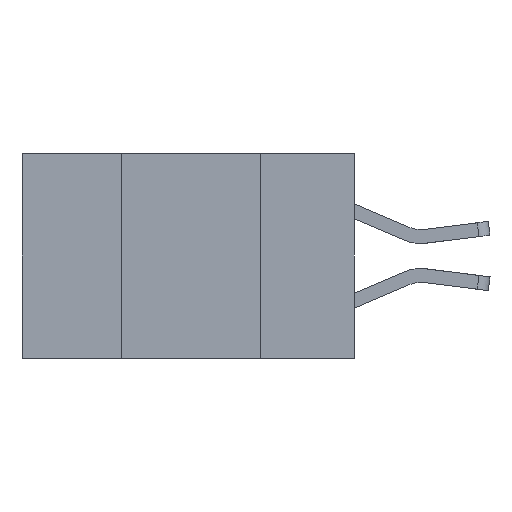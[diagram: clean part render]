
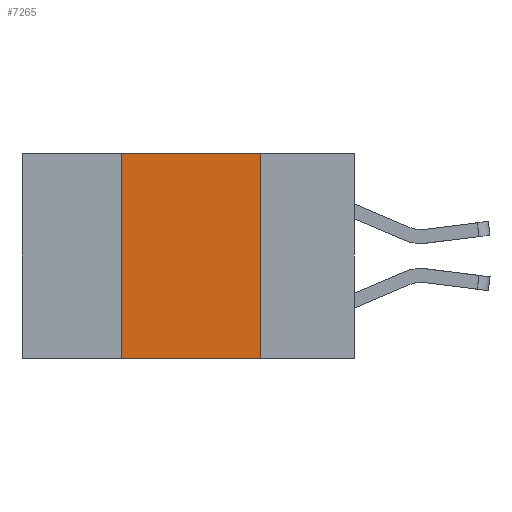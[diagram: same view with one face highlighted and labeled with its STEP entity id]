
A CAD part, left-side view. The second image highlights one B-rep face of the part: STEP entity #7265.
In plain terms, the highlighted planar face has unit normal (-1, 0, 0).
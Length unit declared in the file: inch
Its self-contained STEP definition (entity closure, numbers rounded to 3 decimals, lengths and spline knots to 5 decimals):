
#647 = DIRECTION ( 'NONE',  ( 0., -1., 0. ) ) ;
#957 = EDGE_CURVE ( 'NONE', #5318, #5189, #2652, .T. ) ;
#1039 = PLANE ( 'NONE',  #1068 ) ;
#1068 = AXIS2_PLACEMENT_3D ( 'NONE', #10731, #7375, #2019 ) ;
#1657 = VERTEX_POINT ( 'NONE', #7769 ) ;
#1702 = FACE_OUTER_BOUND ( 'NONE', #4029, .T. ) ;
#1727 = CARTESIAN_POINT ( 'NONE',  ( 0., 0.42, 0. ) ) ;
#1928 = VERTEX_POINT ( 'NONE', #3011 ) ;
#2019 = DIRECTION ( 'NONE',  ( 0., 0., -1. ) ) ;
#2192 = EDGE_CURVE ( 'NONE', #1928, #5189, #9067, .T. ) ;
#2514 = LINE ( 'NONE', #7752, #4333 ) ;
#2652 = LINE ( 'NONE', #10470, #4035 ) ;
#2962 = ORIENTED_EDGE ( 'NONE', *, *, #9389, .F. ) ;
#3011 = CARTESIAN_POINT ( 'NONE',  ( 0., 0.17, 0. ) ) ;
#3498 = DIRECTION ( 'NONE',  ( 0., 0., 1. ) ) ;
#4029 = EDGE_LOOP ( 'NONE', ( #9190, #2962, #11541, #7082 ) ) ;
#4035 = VECTOR ( 'NONE', #8678, 39.37008 ) ;
#4333 = VECTOR ( 'NONE', #647, 39.37008 ) ;
#5189 = VERTEX_POINT ( 'NONE', #11002 ) ;
#5318 = VERTEX_POINT ( 'NONE', #8529 ) ;
#5676 = EDGE_CURVE ( 'NONE', #5318, #1657, #5908, .T. ) ;
#5908 = LINE ( 'NONE', #1727, #10139 ) ;
#6250 = VECTOR ( 'NONE', #7096, 39.37008 ) ;
#7082 = ORIENTED_EDGE ( 'NONE', *, *, #957, .T. ) ;
#7096 = DIRECTION ( 'NONE',  ( 0., 0., -1. ) ) ;
#7265 = ADVANCED_FACE ( 'NONE', ( #1702 ), #1039, .F. ) ;
#7375 = DIRECTION ( 'NONE',  ( 1., 0., 0. ) ) ;
#7752 = CARTESIAN_POINT ( 'NONE',  ( 0., 0.6, 0. ) ) ;
#7769 = CARTESIAN_POINT ( 'NONE',  ( 0., 0.42, 0. ) ) ;
#8529 = CARTESIAN_POINT ( 'NONE',  ( 0., 0.42, -0.37 ) ) ;
#8678 = DIRECTION ( 'NONE',  ( 0., -1., 0. ) ) ;
#8805 = CARTESIAN_POINT ( 'NONE',  ( 0., 0.17, 0. ) ) ;
#9067 = LINE ( 'NONE', #8805, #6250 ) ;
#9190 = ORIENTED_EDGE ( 'NONE', *, *, #2192, .F. ) ;
#9389 = EDGE_CURVE ( 'NONE', #1657, #1928, #2514, .T. ) ;
#10139 = VECTOR ( 'NONE', #3498, 39.37008 ) ;
#10470 = CARTESIAN_POINT ( 'NONE',  ( 0., 0.6, -0.37 ) ) ;
#10731 = CARTESIAN_POINT ( 'NONE',  ( 0., 0.6, 0. ) ) ;
#11002 = CARTESIAN_POINT ( 'NONE',  ( 0., 0.17, -0.37 ) ) ;
#11541 = ORIENTED_EDGE ( 'NONE', *, *, #5676, .F. ) ;
